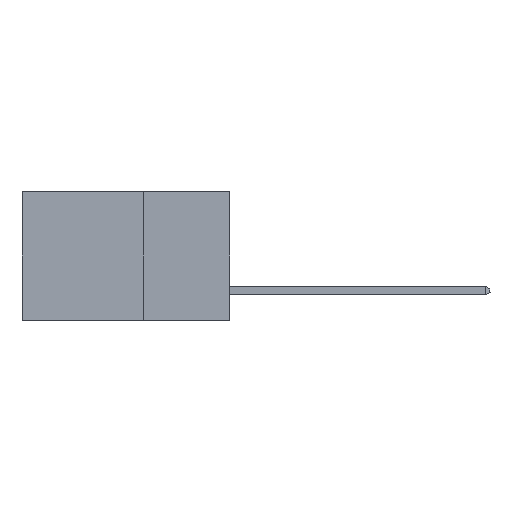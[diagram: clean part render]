
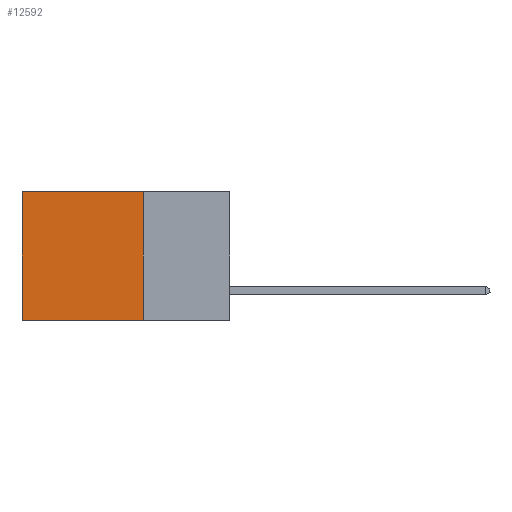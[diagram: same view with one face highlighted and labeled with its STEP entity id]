
A CAD part, left-side view. The second image highlights one B-rep face of the part: STEP entity #12592.
In plain terms, the highlighted planar face has unit normal (-1, 0, 0).
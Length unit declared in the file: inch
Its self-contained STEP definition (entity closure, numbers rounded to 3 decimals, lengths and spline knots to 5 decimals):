
#1102 = ORIENTED_EDGE ( 'NONE', *, *, #17943, .T. ) ;
#2952 = VECTOR ( 'NONE', #8070, 39.37008 ) ;
#3111 = VECTOR ( 'NONE', #16680, 39.37008 ) ;
#3757 = ORIENTED_EDGE ( 'NONE', *, *, #22353, .F. ) ;
#3921 = VERTEX_POINT ( 'NONE', #19219 ) ;
#4545 = ORIENTED_EDGE ( 'NONE', *, *, #8859, .T. ) ;
#4598 = EDGE_CURVE ( 'NONE', #27998, #4970, #26260, .T. ) ;
#4970 = VERTEX_POINT ( 'NONE', #15774 ) ;
#5634 = FACE_OUTER_BOUND ( 'NONE', #17288, .T. ) ;
#5732 = CARTESIAN_POINT ( 'NONE',  ( 0.298, 0.25, 0. ) ) ;
#6746 = VECTOR ( 'NONE', #18474, 39.37008 ) ;
#8070 = DIRECTION ( 'NONE',  ( 0., 0., -1. ) ) ;
#8859 = EDGE_CURVE ( 'NONE', #27998, #11359, #20554, .T. ) ;
#9380 = VECTOR ( 'NONE', #22532, 39.37008 ) ;
#10022 = CARTESIAN_POINT ( 'NONE',  ( 0.298, 0.6, 0. ) ) ;
#11359 = VERTEX_POINT ( 'NONE', #10022 ) ;
#11394 = DIRECTION ( 'NONE',  ( 0., 0., -1. ) ) ;
#12497 = LINE ( 'NONE', #23137, #2952 ) ;
#12592 = ADVANCED_FACE ( 'NONE', ( #5634 ), #26657, .F. ) ;
#12893 = ORIENTED_EDGE ( 'NONE', *, *, #4598, .F. ) ;
#14294 = CARTESIAN_POINT ( 'NONE',  ( 0.298, 0.25, 0. ) ) ;
#15579 = LINE ( 'NONE', #20476, #6746 ) ;
#15774 = CARTESIAN_POINT ( 'NONE',  ( 0.298, 0.25, -0.37 ) ) ;
#16680 = DIRECTION ( 'NONE',  ( 0., 0., -1. ) ) ;
#17288 = EDGE_LOOP ( 'NONE', ( #1102, #3757, #12893, #4545 ) ) ;
#17943 = EDGE_CURVE ( 'NONE', #11359, #3921, #12497, .T. ) ;
#18474 = DIRECTION ( 'NONE',  ( 0., 1., 0. ) ) ;
#19219 = CARTESIAN_POINT ( 'NONE',  ( 0.298, 0.6, -0.37 ) ) ;
#19999 = CARTESIAN_POINT ( 'NONE',  ( 0.298, 0.25, 0. ) ) ;
#20476 = CARTESIAN_POINT ( 'NONE',  ( 0.298, 0.25, -0.37 ) ) ;
#20554 = LINE ( 'NONE', #24829, #9380 ) ;
#22353 = EDGE_CURVE ( 'NONE', #4970, #3921, #15579, .T. ) ;
#22532 = DIRECTION ( 'NONE',  ( 0., 1., 0. ) ) ;
#23137 = CARTESIAN_POINT ( 'NONE',  ( 0.298, 0.6, 0. ) ) ;
#24348 = DIRECTION ( 'NONE',  ( 1., 0., 0. ) ) ;
#24764 = AXIS2_PLACEMENT_3D ( 'NONE', #19999, #24348, #11394 ) ;
#24829 = CARTESIAN_POINT ( 'NONE',  ( 0.298, 0.25, 0. ) ) ;
#26260 = LINE ( 'NONE', #14294, #3111 ) ;
#26657 = PLANE ( 'NONE',  #24764 ) ;
#27998 = VERTEX_POINT ( 'NONE', #5732 ) ;
